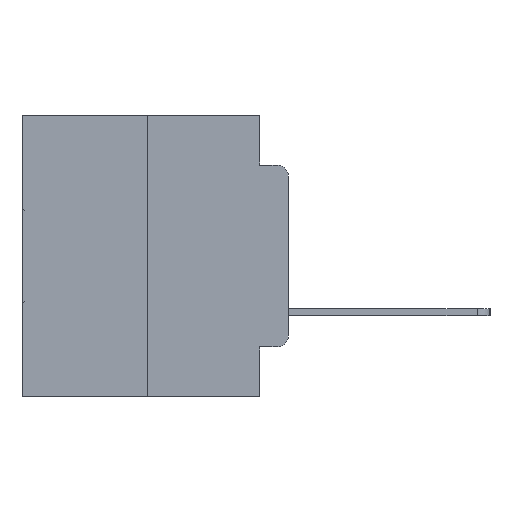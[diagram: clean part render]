
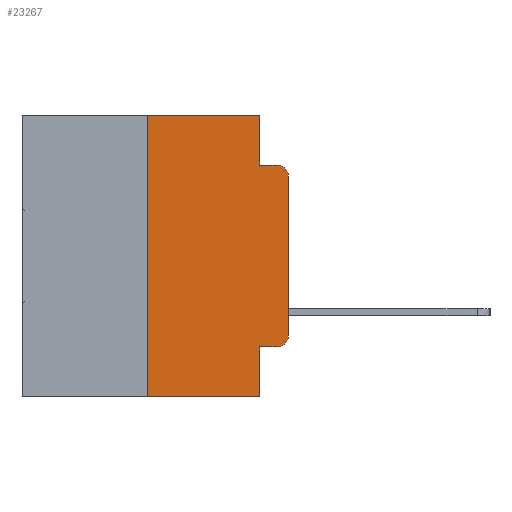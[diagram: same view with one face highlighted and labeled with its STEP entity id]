
A CAD part, left-side view. The second image highlights one B-rep face of the part: STEP entity #23267.
In plain terms, the highlighted planar face has unit normal (-1, 0, 0).
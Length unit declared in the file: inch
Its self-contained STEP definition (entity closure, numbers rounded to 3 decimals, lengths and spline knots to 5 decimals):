
#209 = EDGE_CURVE ( 'NONE', #28592, #11656, #10921, .T. ) ;
#470 = EDGE_LOOP ( 'NONE', ( #1859, #17803, #4013, #14665, #22678, #21984, #18166, #6189, #25427, #12929 ) ) ;
#918 = CARTESIAN_POINT ( 'NONE',  ( 0., 0.02, -0.3915 ) ) ;
#974 = EDGE_CURVE ( 'NONE', #12370, #28592, #7700, .T. ) ;
#1186 = CARTESIAN_POINT ( 'NONE',  ( 0., 0.051, 0. ) ) ;
#1720 = CIRCLE ( 'NONE', #20049, 0.02 ) ;
#1859 = ORIENTED_EDGE ( 'NONE', *, *, #974, .T. ) ;
#2086 = VERTEX_POINT ( 'NONE', #1186 ) ;
#2935 = CARTESIAN_POINT ( 'NONE',  ( 0., 0.051, -0.4115 ) ) ;
#3266 = DIRECTION ( 'NONE',  ( 0., 0., -1. ) ) ;
#3669 = LINE ( 'NONE', #22930, #13627 ) ;
#3952 = EDGE_CURVE ( 'NONE', #15722, #2086, #11514, .T. ) ;
#4013 = ORIENTED_EDGE ( 'NONE', *, *, #8952, .F. ) ;
#4347 = DIRECTION ( 'NONE',  ( 0., 0., -1. ) ) ;
#4436 = LINE ( 'NONE', #25625, #17194 ) ;
#4884 = DIRECTION ( 'NONE',  ( 0., -1., 0. ) ) ;
#5154 = CARTESIAN_POINT ( 'NONE',  ( 0., 0.051, 0. ) ) ;
#5658 = LINE ( 'NONE', #2935, #10995 ) ;
#5849 = EDGE_CURVE ( 'NONE', #26339, #12370, #1720, .T. ) ;
#6189 = ORIENTED_EDGE ( 'NONE', *, *, #26450, .F. ) ;
#6437 = EDGE_CURVE ( 'NONE', #11084, #26339, #5658, .T. ) ;
#6591 = CARTESIAN_POINT ( 'NONE',  ( 0., 0.051, 0. ) ) ;
#7123 = PLANE ( 'NONE',  #20011 ) ;
#7371 = DIRECTION ( 'NONE',  ( 0., 0., 1. ) ) ;
#7428 = CARTESIAN_POINT ( 'NONE',  ( 0., 0., 0. ) ) ;
#7700 = LINE ( 'NONE', #7428, #26179 ) ;
#7980 = CARTESIAN_POINT ( 'NONE',  ( 0., 0., -0.1085 ) ) ;
#8696 = VERTEX_POINT ( 'NONE', #26338 ) ;
#8952 = EDGE_CURVE ( 'NONE', #18767, #11656, #24610, .T. ) ;
#9428 = CARTESIAN_POINT ( 'NONE',  ( 0., 0.473, 0. ) ) ;
#9533 = DIRECTION ( 'NONE',  ( 0., 0., -1. ) ) ;
#10812 = CARTESIAN_POINT ( 'NONE',  ( 0., 0., -0.3915 ) ) ;
#10921 = CIRCLE ( 'NONE', #16664, 0.02 ) ;
#10995 = VECTOR ( 'NONE', #16500, 39.37008 ) ;
#11084 = VERTEX_POINT ( 'NONE', #17521 ) ;
#11336 = DIRECTION ( 'NONE',  ( 0., -1., 0. ) ) ;
#11514 = LINE ( 'NONE', #24552, #22666 ) ;
#11656 = VERTEX_POINT ( 'NONE', #26205 ) ;
#11677 = DIRECTION ( 'NONE',  ( 1., 0., 0. ) ) ;
#12370 = VERTEX_POINT ( 'NONE', #10812 ) ;
#12929 = ORIENTED_EDGE ( 'NONE', *, *, #5849, .T. ) ;
#13296 = VERTEX_POINT ( 'NONE', #14586 ) ;
#13436 = LINE ( 'NONE', #5154, #24543 ) ;
#13627 = VECTOR ( 'NONE', #16301, 39.37008 ) ;
#14194 = VECTOR ( 'NONE', #4884, 39.37008 ) ;
#14586 = CARTESIAN_POINT ( 'NONE',  ( 0., 0.25, -0.5 ) ) ;
#14665 = ORIENTED_EDGE ( 'NONE', *, *, #19437, .F. ) ;
#15226 = FACE_OUTER_BOUND ( 'NONE', #470, .T. ) ;
#15722 = VERTEX_POINT ( 'NONE', #29063 ) ;
#16159 = CARTESIAN_POINT ( 'NONE',  ( 0., 0.051, -0.0885 ) ) ;
#16301 = DIRECTION ( 'NONE',  ( 0., 0., 1. ) ) ;
#16500 = DIRECTION ( 'NONE',  ( 0., -1., 0. ) ) ;
#16664 = AXIS2_PLACEMENT_3D ( 'NONE', #18232, #19889, #9533 ) ;
#16834 = DIRECTION ( 'NONE',  ( -1., 0., 0. ) ) ;
#17194 = VECTOR ( 'NONE', #19067, 39.37008 ) ;
#17521 = CARTESIAN_POINT ( 'NONE',  ( 0., 0.051, -0.4115 ) ) ;
#17803 = ORIENTED_EDGE ( 'NONE', *, *, #209, .T. ) ;
#18166 = ORIENTED_EDGE ( 'NONE', *, *, #20408, .T. ) ;
#18232 = CARTESIAN_POINT ( 'NONE',  ( 0., 0.02, -0.1085 ) ) ;
#18667 = DIRECTION ( 'NONE',  ( 0., 0., -1. ) ) ;
#18767 = VERTEX_POINT ( 'NONE', #28270 ) ;
#19067 = DIRECTION ( 'NONE',  ( 0., -1., 0. ) ) ;
#19341 = VECTOR ( 'NONE', #4347, 39.37008 ) ;
#19437 = EDGE_CURVE ( 'NONE', #2086, #18767, #25213, .T. ) ;
#19889 = DIRECTION ( 'NONE',  ( -1., 0., 0. ) ) ;
#20011 = AXIS2_PLACEMENT_3D ( 'NONE', #9428, #11677, #27203 ) ;
#20049 = AXIS2_PLACEMENT_3D ( 'NONE', #918, #16834, #3266 ) ;
#20408 = EDGE_CURVE ( 'NONE', #13296, #8696, #4436, .T. ) ;
#20503 = CARTESIAN_POINT ( 'NONE',  ( 0., 0.02, -0.4115 ) ) ;
#20919 = EDGE_CURVE ( 'NONE', #13296, #15722, #3669, .T. ) ;
#21984 = ORIENTED_EDGE ( 'NONE', *, *, #20919, .F. ) ;
#22666 = VECTOR ( 'NONE', #11336, 39.37008 ) ;
#22678 = ORIENTED_EDGE ( 'NONE', *, *, #3952, .F. ) ;
#22930 = CARTESIAN_POINT ( 'NONE',  ( 0., 0.25, 0. ) ) ;
#23267 = ADVANCED_FACE ( 'NONE', ( #15226 ), #7123, .F. ) ;
#24543 = VECTOR ( 'NONE', #18667, 39.37008 ) ;
#24552 = CARTESIAN_POINT ( 'NONE',  ( 0., 0.473, 0. ) ) ;
#24610 = LINE ( 'NONE', #16159, #14194 ) ;
#25213 = LINE ( 'NONE', #6591, #19341 ) ;
#25427 = ORIENTED_EDGE ( 'NONE', *, *, #6437, .T. ) ;
#25625 = CARTESIAN_POINT ( 'NONE',  ( 0., 0.473, -0.5 ) ) ;
#26179 = VECTOR ( 'NONE', #7371, 39.37008 ) ;
#26205 = CARTESIAN_POINT ( 'NONE',  ( 0., 0.02, -0.0885 ) ) ;
#26338 = CARTESIAN_POINT ( 'NONE',  ( 0., 0.051, -0.5 ) ) ;
#26339 = VERTEX_POINT ( 'NONE', #20503 ) ;
#26450 = EDGE_CURVE ( 'NONE', #11084, #8696, #13436, .T. ) ;
#27203 = DIRECTION ( 'NONE',  ( 0., 0., -1. ) ) ;
#28270 = CARTESIAN_POINT ( 'NONE',  ( 0., 0.051, -0.0885 ) ) ;
#28592 = VERTEX_POINT ( 'NONE', #7980 ) ;
#29063 = CARTESIAN_POINT ( 'NONE',  ( 0., 0.25, 0. ) ) ;
